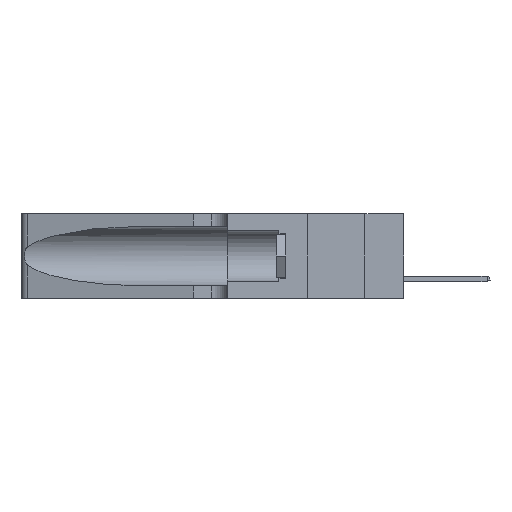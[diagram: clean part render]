
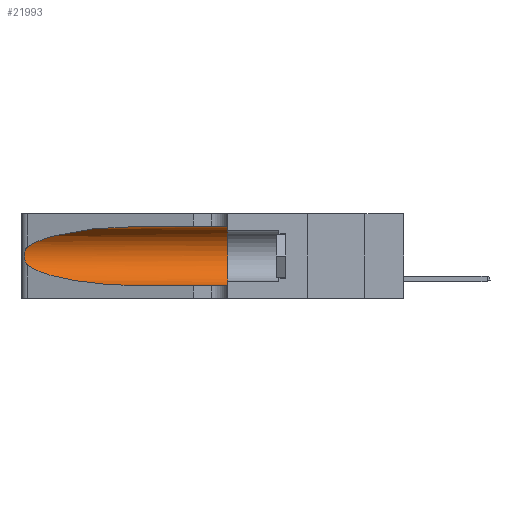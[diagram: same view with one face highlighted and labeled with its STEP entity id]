
A CAD part, left-side view. The second image highlights one B-rep face of the part: STEP entity #21993.
In plain terms, the highlighted cylindrical face has radius 3.308 mm (diameter 6.617 mm), a partial arc.
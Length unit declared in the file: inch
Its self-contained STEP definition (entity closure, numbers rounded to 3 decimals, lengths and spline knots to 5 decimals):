
#5 = CIRCLE ( 'NONE', #22922, 0.13025 ) ;
#44 = DIRECTION ( 'NONE',  ( 0., 0., 1. ) ) ;
#295 = CARTESIAN_POINT ( 'NONE',  ( 0.25639, 1.23184, 0.21858 ) ) ;
#501 = VERTEX_POINT ( 'NONE', #14007 ) ;
#694 = CARTESIAN_POINT ( 'NONE',  ( 0.1305, 0.35, 0.05475 ) ) ;
#923 = CARTESIAN_POINT ( 'NONE',  ( 0.25856, 1.23593, 0.16098 ) ) ;
#1167 = CARTESIAN_POINT ( 'NONE',  ( 0.1305, 0.72297, 0.05475 ) ) ;
#1308 = CARTESIAN_POINT ( 'NONE',  ( 0.1305, 0.72297, 0.31525 ) ) ;
#2008 = ORIENTED_EDGE ( 'NONE', *, *, #19772, .F. ) ;
#2065 = EDGE_CURVE ( 'NONE', #12456, #19333, #20175, .T. ) ;
#2379 = CARTESIAN_POINT ( 'NONE',  ( 0.26075, 1.23896, 0.178 ) ) ;
#3162 = CARTESIAN_POINT ( 'NONE',  ( 0.18966, 0.96281, 0.31525 ) ) ;
#3169 = AXIS2_PLACEMENT_3D ( 'NONE', #8436, #4795, #6516 ) ;
#3485 = VERTEX_POINT ( 'NONE', #16181 ) ;
#3538 = CARTESIAN_POINT ( 'NONE',  ( 0.1305, 1.61858, 0.05475 ) ) ;
#4056 = CARTESIAN_POINT ( 'NONE',  ( 0.25854, 1.2359, 0.20912 ) ) ;
#4795 = DIRECTION ( 'NONE',  ( 0., -1., 0. ) ) ;
#4932 = ORIENTED_EDGE ( 'NONE', *, *, #16993, .T. ) ;
#5123 = EDGE_LOOP ( 'NONE', ( #4932, #23345, #6958, #6484, #2008, #19087 ) ) ;
#6323 = CARTESIAN_POINT ( 'NONE',  ( 0.26017, 1.23833, 0.17102 ) ) ;
#6484 = ORIENTED_EDGE ( 'NONE', *, *, #2065, .T. ) ;
#6516 = DIRECTION ( 'NONE',  ( 0., 0., -1. ) ) ;
#6703 = CARTESIAN_POINT ( 'NONE',  ( 0.1305, 0.72297, 0.31525 ) ) ;
#6958 = ORIENTED_EDGE ( 'NONE', *, *, #12729, .T. ) ;
#7273 = EDGE_CURVE ( 'NONE', #20158, #3485, #8028, .T. ) ;
#7343 = CARTESIAN_POINT ( 'NONE',  ( 0.18966, 0.96281, 0.05475 ) ) ;
#8028 = B_SPLINE_CURVE_WITH_KNOTS ( 'NONE', 3,
 ( #10261, #11156, #295, #9505, #4056, #11306, #18568, #2379, #6323, #923, #11907, #19457, #20641, #8434 ),
 .UNSPECIFIED., .F., .F.,
 ( 4, 2, 2, 2, 2, 2, 4 ),
 ( 0., 0.00027, 0.00053, 0.00107, 0.0016, 0.00187, 0.00214 ),
 .UNSPECIFIED. ) ;
#8434 = CARTESIAN_POINT ( 'NONE',  ( 0.25487, 1.22718, 0.14631 ) ) ;
#8436 = CARTESIAN_POINT ( 'NONE',  ( 0.1305, 1.61858, 0.185 ) ) ;
#9505 = CARTESIAN_POINT ( 'NONE',  ( 0.25787, 1.23484, 0.2124 ) ) ;
#10261 = CARTESIAN_POINT ( 'NONE',  ( 0.25487, 1.22718, 0.22369 ) ) ;
#10560 = DIRECTION ( 'NONE',  ( 0., -1., 0. ) ) ;
#10571 = CARTESIAN_POINT ( 'NONE',  ( 0.25487, 1.22718, 0.22369 ) ) ;
#10637 = CARTESIAN_POINT ( 'NONE',  ( 0.25487, 1.22718, 0.22369 ) ) ;
#10740 = CARTESIAN_POINT ( 'NONE',  ( 0.1305, 0.35, 0.185 ) ) ;
#10779 = FACE_OUTER_BOUND ( 'NONE', #5123, .T. ) ;
#11156 = CARTESIAN_POINT ( 'NONE',  ( 0.25555, 1.22994, 0.2215 ) ) ;
#11306 = CARTESIAN_POINT ( 'NONE',  ( 0.26018, 1.23835, 0.19895 ) ) ;
#11498 =( BOUNDED_CURVE ( )  B_SPLINE_CURVE ( 3, ( #14517, #17974, #7343, #16527 ),
 .UNSPECIFIED., .F., .F. ) 
 B_SPLINE_CURVE_WITH_KNOTS ( ( 4, 4 ),
 ( 3.44316, 4.71239 ),
 .UNSPECIFIED. ) 
 CURVE ( )  GEOMETRIC_REPRESENTATION_ITEM ( )  RATIONAL_B_SPLINE_CURVE ( ( 1., 0.87, 0.87, 1. ) ) 
 REPRESENTATION_ITEM ( '' )  );
#11907 = CARTESIAN_POINT ( 'NONE',  ( 0.25789, 1.23486, 0.15765 ) ) ;
#12456 = VERTEX_POINT ( 'NONE', #1167 ) ;
#12729 = EDGE_CURVE ( 'NONE', #3485, #12456, #11498, .T. ) ;
#14007 = CARTESIAN_POINT ( 'NONE',  ( 0.1305, 0.35, 0.31525 ) ) ;
#14517 = CARTESIAN_POINT ( 'NONE',  ( 0.25487, 1.22718, 0.14631 ) ) ;
#15038 = CYLINDRICAL_SURFACE ( 'NONE', #3169, 0.13025 ) ;
#15793 = CARTESIAN_POINT ( 'NONE',  ( 0.2373, 1.15595, 0.28018 ) ) ;
#15995 = VERTEX_POINT ( 'NONE', #6703 ) ;
#16181 = CARTESIAN_POINT ( 'NONE',  ( 0.25487, 1.22718, 0.14631 ) ) ;
#16188 = DIRECTION ( 'NONE',  ( 0., -1., 0. ) ) ;
#16527 = CARTESIAN_POINT ( 'NONE',  ( 0.1305, 0.72297, 0.05475 ) ) ;
#16562 = VECTOR ( 'NONE', #16188, 39.37008 ) ;
#16993 = EDGE_CURVE ( 'NONE', #15995, #20158, #18120, .T. ) ;
#17974 = CARTESIAN_POINT ( 'NONE',  ( 0.2373, 1.15595, 0.08982 ) ) ;
#18120 =( BOUNDED_CURVE ( )  B_SPLINE_CURVE ( 3, ( #1308, #3162, #15793, #10571 ),
 .UNSPECIFIED., .F., .F. ) 
 B_SPLINE_CURVE_WITH_KNOTS ( ( 4, 4 ),
 ( 1.5708, 2.84003 ),
 .UNSPECIFIED. ) 
 CURVE ( )  GEOMETRIC_REPRESENTATION_ITEM ( )  RATIONAL_B_SPLINE_CURVE ( ( 1., 0.87, 0.87, 1. ) ) 
 REPRESENTATION_ITEM ( '' )  );
#18164 = LINE ( 'NONE', #23410, #22422 ) ;
#18568 = CARTESIAN_POINT ( 'NONE',  ( 0.26075, 1.23896, 0.19203 ) ) ;
#19087 = ORIENTED_EDGE ( 'NONE', *, *, #21271, .F. ) ;
#19333 = VERTEX_POINT ( 'NONE', #694 ) ;
#19457 = CARTESIAN_POINT ( 'NONE',  ( 0.25639, 1.23186, 0.15144 ) ) ;
#19772 = EDGE_CURVE ( 'NONE', #501, #19333, #5, .T. ) ;
#20158 = VERTEX_POINT ( 'NONE', #10637 ) ;
#20175 = LINE ( 'NONE', #3538, #16562 ) ;
#20641 = CARTESIAN_POINT ( 'NONE',  ( 0.25555, 1.22993, 0.14849 ) ) ;
#21271 = EDGE_CURVE ( 'NONE', #15995, #501, #18164, .T. ) ;
#21461 = DIRECTION ( 'NONE',  ( 0., 1., 0. ) ) ;
#21993 = ADVANCED_FACE ( 'NONE', ( #10779 ), #15038, .F. ) ;
#22422 = VECTOR ( 'NONE', #10560, 39.37008 ) ;
#22922 = AXIS2_PLACEMENT_3D ( 'NONE', #10740, #21461, #44 ) ;
#23345 = ORIENTED_EDGE ( 'NONE', *, *, #7273, .T. ) ;
#23410 = CARTESIAN_POINT ( 'NONE',  ( 0.1305, 1.61858, 0.31525 ) ) ;
